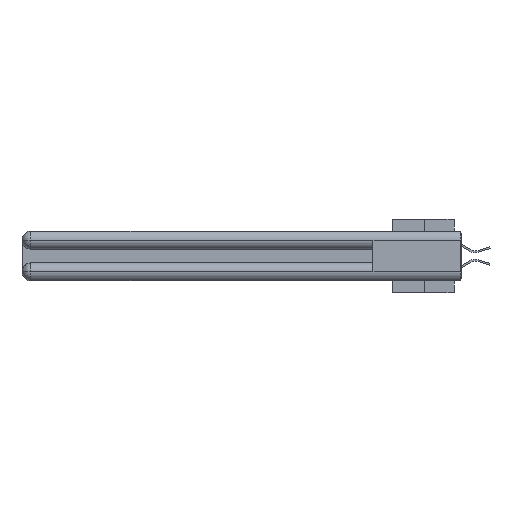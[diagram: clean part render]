
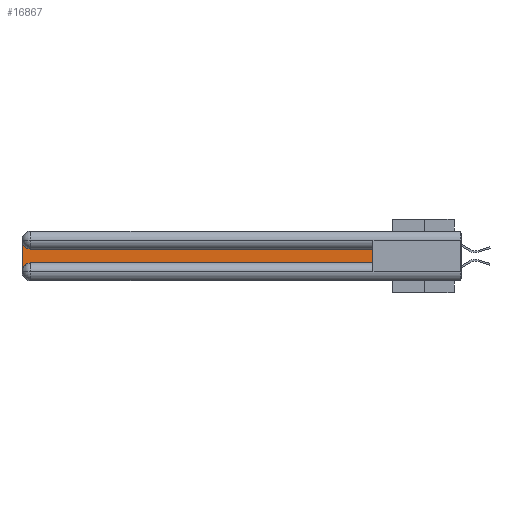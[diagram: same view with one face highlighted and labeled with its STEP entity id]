
A CAD part, left-side view. The second image highlights one B-rep face of the part: STEP entity #16867.
In plain terms, the highlighted planar face has unit normal (-1, 0, 0).
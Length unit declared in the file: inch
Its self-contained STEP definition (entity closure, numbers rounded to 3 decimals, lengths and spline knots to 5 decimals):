
#140 = DIRECTION ( 'NONE',  ( 1., 0., 0. ) ) ;
#1021 = ORIENTED_EDGE ( 'NONE', *, *, #19464, .T. ) ;
#1478 = CIRCLE ( 'NONE', #20713, 0.06 ) ;
#2058 = DIRECTION ( 'NONE',  ( 0., -1., 0. ) ) ;
#2866 = EDGE_CURVE ( 'NONE', #15829, #28595, #30400, .T. ) ;
#3784 = ORIENTED_EDGE ( 'NONE', *, *, #10950, .T. ) ;
#4438 = DIRECTION ( 'NONE',  ( 0., 0., -1. ) ) ;
#4718 = EDGE_CURVE ( 'NONE', #9646, #23887, #15100, .T. ) ;
#5656 = FACE_OUTER_BOUND ( 'NONE', #11003, .T. ) ;
#6688 = ORIENTED_EDGE ( 'NONE', *, *, #4718, .T. ) ;
#7187 = VERTEX_POINT ( 'NONE', #16593 ) ;
#7747 = LINE ( 'NONE', #12752, #18372 ) ;
#8178 = CARTESIAN_POINT ( 'NONE',  ( 0.075, 2.94, -0.2175 ) ) ;
#9646 = VERTEX_POINT ( 'NONE', #30593 ) ;
#9664 = CARTESIAN_POINT ( 'NONE',  ( 0.075, 2.94, -0.1225 ) ) ;
#10950 = EDGE_CURVE ( 'NONE', #28595, #26080, #23694, .T. ) ;
#11003 = EDGE_LOOP ( 'NONE', ( #6688, #1021, #31232, #3784, #30455, #24340 ) ) ;
#11148 = EDGE_CURVE ( 'NONE', #7187, #9646, #33485, .T. ) ;
#11173 = CARTESIAN_POINT ( 'NONE',  ( 0.075, 2.94, -0.2775 ) ) ;
#12115 = DIRECTION ( 'NONE',  ( 0., 0., -1. ) ) ;
#12752 = CARTESIAN_POINT ( 'NONE',  ( 0.075, 0.6, -0.2175 ) ) ;
#12818 = AXIS2_PLACEMENT_3D ( 'NONE', #11173, #28881, #23713 ) ;
#13097 = DIRECTION ( 'NONE',  ( 0., 0., -1. ) ) ;
#15100 = LINE ( 'NONE', #25565, #29958 ) ;
#15829 = VERTEX_POINT ( 'NONE', #27834 ) ;
#16160 = PLANE ( 'NONE',  #33186 ) ;
#16593 = CARTESIAN_POINT ( 'NONE',  ( 0.075, 0.6, -0.2175 ) ) ;
#16867 = ADVANCED_FACE ( 'NONE', ( #5656 ), #16160, .F. ) ;
#17525 = CARTESIAN_POINT ( 'NONE',  ( 0.075, 3., -0.2175 ) ) ;
#18372 = VECTOR ( 'NONE', #2058, 39.37008 ) ;
#19464 = EDGE_CURVE ( 'NONE', #23887, #15829, #1478, .T. ) ;
#20010 = VECTOR ( 'NONE', #4438, 39.37008 ) ;
#20713 = AXIS2_PLACEMENT_3D ( 'NONE', #26892, #30309, #12115 ) ;
#20815 = CARTESIAN_POINT ( 'NONE',  ( 0.075, 3., -0.1225 ) ) ;
#23694 = CIRCLE ( 'NONE', #12818, 0.06 ) ;
#23713 = DIRECTION ( 'NONE',  ( 0., 0., -1. ) ) ;
#23797 = EDGE_CURVE ( 'NONE', #26080, #7187, #7747, .T. ) ;
#23887 = VERTEX_POINT ( 'NONE', #9664 ) ;
#24340 = ORIENTED_EDGE ( 'NONE', *, *, #11148, .T. ) ;
#25341 = CARTESIAN_POINT ( 'NONE',  ( 0.075, 3., -0.2775 ) ) ;
#25565 = CARTESIAN_POINT ( 'NONE',  ( 0.075, 0.6, -0.1225 ) ) ;
#26080 = VERTEX_POINT ( 'NONE', #8178 ) ;
#26892 = CARTESIAN_POINT ( 'NONE',  ( 0.075, 2.94, -0.0625 ) ) ;
#27834 = CARTESIAN_POINT ( 'NONE',  ( 0.075, 3., -0.0625 ) ) ;
#28504 = DIRECTION ( 'NONE',  ( 0., 0., 1. ) ) ;
#28595 = VERTEX_POINT ( 'NONE', #25341 ) ;
#28881 = DIRECTION ( 'NONE',  ( 1., 0., 0. ) ) ;
#29958 = VECTOR ( 'NONE', #33112, 39.37008 ) ;
#30309 = DIRECTION ( 'NONE',  ( 1., 0., 0. ) ) ;
#30400 = LINE ( 'NONE', #17525, #20010 ) ;
#30455 = ORIENTED_EDGE ( 'NONE', *, *, #23797, .T. ) ;
#30593 = CARTESIAN_POINT ( 'NONE',  ( 0.075, 0.6, -0.1225 ) ) ;
#31232 = ORIENTED_EDGE ( 'NONE', *, *, #2866, .T. ) ;
#32968 = CARTESIAN_POINT ( 'NONE',  ( 0.075, 0.6, -0.2175 ) ) ;
#33112 = DIRECTION ( 'NONE',  ( 0., 1., 0. ) ) ;
#33186 = AXIS2_PLACEMENT_3D ( 'NONE', #20815, #140, #13097 ) ;
#33485 = LINE ( 'NONE', #32968, #33628 ) ;
#33628 = VECTOR ( 'NONE', #28504, 39.37008 ) ;
